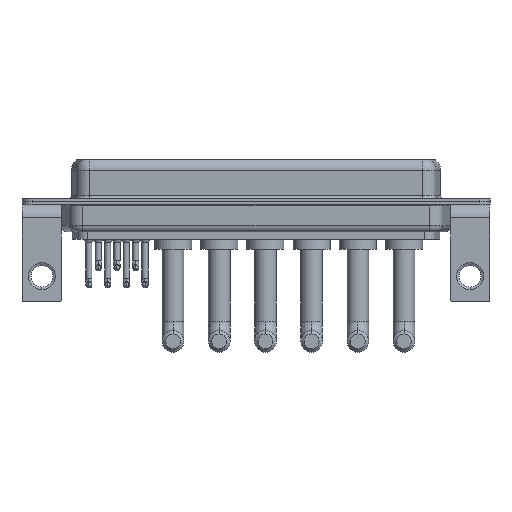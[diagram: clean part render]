
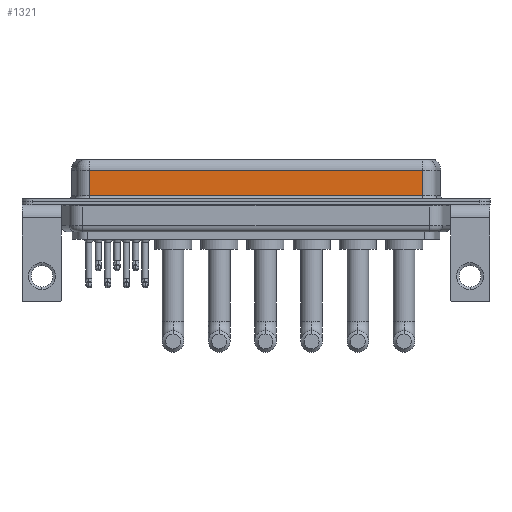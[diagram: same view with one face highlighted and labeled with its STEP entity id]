
A CAD part, front view. The second image highlights one B-rep face of the part: STEP entity #1321.
In plain terms, the highlighted planar face has unit normal (0, -1, 0).
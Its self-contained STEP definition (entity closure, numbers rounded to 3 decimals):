
#775 = DIRECTION ( 'NONE',  ( 0., 0., 1. ) ) ;
#1297 = DIRECTION ( 'NONE',  ( 0., 0., -1. ) ) ;
#1321 = ADVANCED_FACE ( 'NONE', ( #11078 ), #12725, .F. ) ;
#2532 = VECTOR ( 'NONE', #17739, 1000. ) ;
#2904 = CARTESIAN_POINT ( 'NONE',  ( 7.038, -3.95, 0.9 ) ) ;
#3370 = EDGE_CURVE ( 'NONE', #6729, #18532, #16494, .T. ) ;
#3409 = EDGE_CURVE ( 'NONE', #10046, #10817, #13616, .T. ) ;
#3607 = ORIENTED_EDGE ( 'NONE', *, *, #6636, .F. ) ;
#4079 = CARTESIAN_POINT ( 'NONE',  ( 56.462, -3.95, 4.65 ) ) ;
#4670 = DIRECTION ( 'NONE',  ( 1., 0., 0. ) ) ;
#5779 = EDGE_CURVE ( 'NONE', #10817, #6729, #11779, .T. ) ;
#6542 = VECTOR ( 'NONE', #1297, 1000. ) ;
#6636 = EDGE_CURVE ( 'NONE', #10046, #18532, #11834, .T. ) ;
#6729 = VERTEX_POINT ( 'NONE', #2904 ) ;
#7120 = CARTESIAN_POINT ( 'NONE',  ( 7.038, -3.95, 4.65 ) ) ;
#7871 = DIRECTION ( 'NONE',  ( -1., 0., 0. ) ) ;
#8214 = ORIENTED_EDGE ( 'NONE', *, *, #5779, .T. ) ;
#9615 = CARTESIAN_POINT ( 'NONE',  ( 56.462, -3.95, 6.4 ) ) ;
#9822 = AXIS2_PLACEMENT_3D ( 'NONE', #9615, #12179, #775 ) ;
#10046 = VERTEX_POINT ( 'NONE', #4079 ) ;
#10101 = CARTESIAN_POINT ( 'NONE',  ( 56.462, -3.95, 6.4 ) ) ;
#10783 = CARTESIAN_POINT ( 'NONE',  ( 56.462, -3.95, 0.9 ) ) ;
#10817 = VERTEX_POINT ( 'NONE', #7120 ) ;
#11078 = FACE_OUTER_BOUND ( 'NONE', #17010, .T. ) ;
#11779 = LINE ( 'NONE', #16239, #6542 ) ;
#11834 = LINE ( 'NONE', #10101, #2532 ) ;
#12142 = CARTESIAN_POINT ( 'NONE',  ( 56.462, -3.95, 4.65 ) ) ;
#12179 = DIRECTION ( 'NONE',  ( 0., 1., 0. ) ) ;
#12432 = ORIENTED_EDGE ( 'NONE', *, *, #3409, .T. ) ;
#12725 = PLANE ( 'NONE',  #9822 ) ;
#13374 = CARTESIAN_POINT ( 'NONE',  ( 56.462, -3.95, 0.9 ) ) ;
#13616 = LINE ( 'NONE', #12142, #16434 ) ;
#16239 = CARTESIAN_POINT ( 'NONE',  ( 7.038, -3.95, 6.4 ) ) ;
#16434 = VECTOR ( 'NONE', #7871, 1000. ) ;
#16494 = LINE ( 'NONE', #10783, #18596 ) ;
#17010 = EDGE_LOOP ( 'NONE', ( #3607, #12432, #8214, #18069 ) ) ;
#17739 = DIRECTION ( 'NONE',  ( 0., 0., -1. ) ) ;
#18069 = ORIENTED_EDGE ( 'NONE', *, *, #3370, .T. ) ;
#18532 = VERTEX_POINT ( 'NONE', #13374 ) ;
#18596 = VECTOR ( 'NONE', #4670, 1000. ) ;
